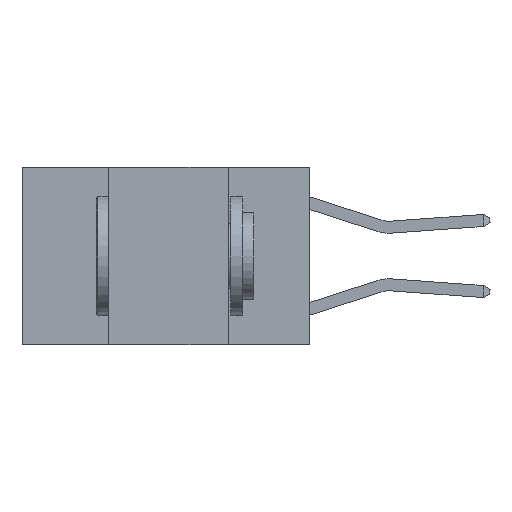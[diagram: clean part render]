
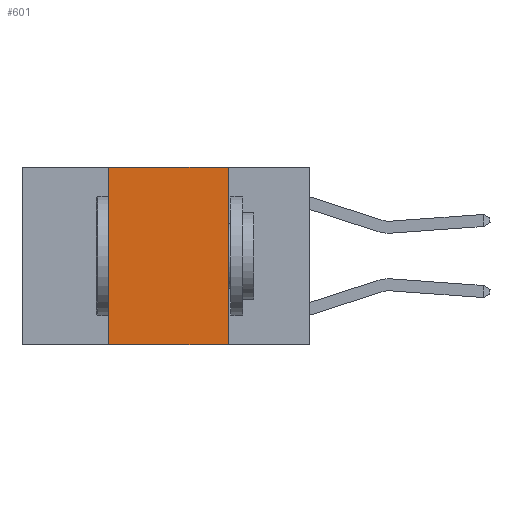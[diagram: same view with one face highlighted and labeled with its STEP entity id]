
A CAD part, left-side view. The second image highlights one B-rep face of the part: STEP entity #601.
In plain terms, the highlighted planar face has unit normal (-1, 0, 0).
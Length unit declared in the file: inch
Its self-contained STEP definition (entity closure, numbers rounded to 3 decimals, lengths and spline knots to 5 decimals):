
#601 = ADVANCED_FACE ( 'NONE', ( #902 ), #10725, .F. ) ;
#717 = VECTOR ( 'NONE', #11307, 39.37008 ) ;
#902 = FACE_OUTER_BOUND ( 'NONE', #6958, .T. ) ;
#1379 = LINE ( 'NONE', #27163, #13636 ) ;
#4614 = VERTEX_POINT ( 'NONE', #17756 ) ;
#5523 = VERTEX_POINT ( 'NONE', #10632 ) ;
#6958 = EDGE_LOOP ( 'NONE', ( #12298, #13437, #22540, #27852 ) ) ;
#7097 = CARTESIAN_POINT ( 'NONE',  ( 0., 0.17, 0. ) ) ;
#7434 = EDGE_CURVE ( 'NONE', #22140, #24774, #19374, .T. ) ;
#9997 = LINE ( 'NONE', #7097, #25101 ) ;
#10632 = CARTESIAN_POINT ( 'NONE',  ( 0., 0.17, -0.37 ) ) ;
#10725 = PLANE ( 'NONE',  #27816 ) ;
#11307 = DIRECTION ( 'NONE',  ( 0., 0., 1. ) ) ;
#11758 = CARTESIAN_POINT ( 'NONE',  ( 0., 0.42, 0. ) ) ;
#12298 = ORIENTED_EDGE ( 'NONE', *, *, #12871, .F. ) ;
#12553 = DIRECTION ( 'NONE',  ( 0., 0., -1. ) ) ;
#12871 = EDGE_CURVE ( 'NONE', #24774, #5523, #9997, .T. ) ;
#13437 = ORIENTED_EDGE ( 'NONE', *, *, #7434, .F. ) ;
#13636 = VECTOR ( 'NONE', #17958, 39.37008 ) ;
#16184 = EDGE_CURVE ( 'NONE', #4614, #22140, #20667, .T. ) ;
#17756 = CARTESIAN_POINT ( 'NONE',  ( 0., 0.42, -0.37 ) ) ;
#17958 = DIRECTION ( 'NONE',  ( 0., -1., 0. ) ) ;
#19374 = LINE ( 'NONE', #19675, #22097 ) ;
#19675 = CARTESIAN_POINT ( 'NONE',  ( 0., 0.6, 0. ) ) ;
#20667 = LINE ( 'NONE', #11758, #717 ) ;
#21452 = EDGE_CURVE ( 'NONE', #4614, #5523, #1379, .T. ) ;
#22097 = VECTOR ( 'NONE', #28725, 39.37008 ) ;
#22140 = VERTEX_POINT ( 'NONE', #28472 ) ;
#22540 = ORIENTED_EDGE ( 'NONE', *, *, #16184, .F. ) ;
#24221 = CARTESIAN_POINT ( 'NONE',  ( 0., 0.17, 0. ) ) ;
#24539 = DIRECTION ( 'NONE',  ( 1., 0., 0. ) ) ;
#24774 = VERTEX_POINT ( 'NONE', #24221 ) ;
#25101 = VECTOR ( 'NONE', #28558, 39.37008 ) ;
#27163 = CARTESIAN_POINT ( 'NONE',  ( 0., 0.6, -0.37 ) ) ;
#27816 = AXIS2_PLACEMENT_3D ( 'NONE', #29286, #24539, #12553 ) ;
#27852 = ORIENTED_EDGE ( 'NONE', *, *, #21452, .T. ) ;
#28472 = CARTESIAN_POINT ( 'NONE',  ( 0., 0.42, 0. ) ) ;
#28558 = DIRECTION ( 'NONE',  ( 0., 0., -1. ) ) ;
#28725 = DIRECTION ( 'NONE',  ( 0., -1., 0. ) ) ;
#29286 = CARTESIAN_POINT ( 'NONE',  ( 0., 0.6, 0. ) ) ;
